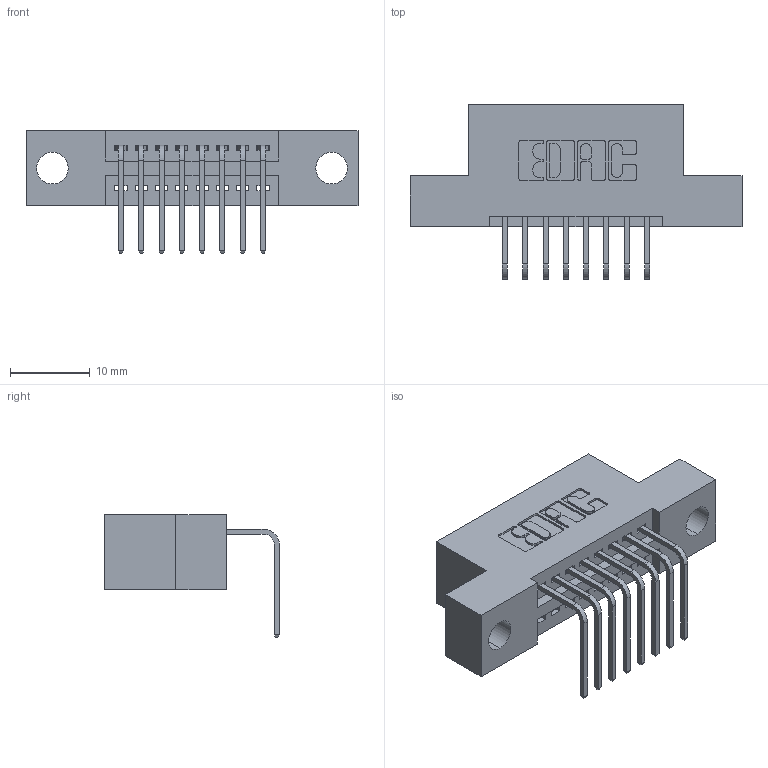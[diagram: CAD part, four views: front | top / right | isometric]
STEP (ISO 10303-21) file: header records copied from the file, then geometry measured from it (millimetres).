
FILE_DESCRIPTION (( 'STEP AP203' ), '1' );
FILE_NAME ('345-008-558-104.STEP', '2021-06-01T16:09:02', ( '' ), ( '' ), 'SwSTEP 2.0', 'SolidWorks 2020', '' );
FILE_SCHEMA (( 'CONFIG_CONTROL_DESIGN' ));
Length unit declared in the file: inch
Products named in the file (3): 345-008-558-104; 345-292-001_558 Tail - 2; 345 Part_Flush Mounting Lugs - 0.156 Dia-TI
Assembly tree (9 placements, depth 2):
  345-008-558-104
    345 Part_Flush Mounting Lugs - 0.156 Dia-TI
    345-292-001_558 Tail - 2  x8
Bounding box: 41.53 x 21.83 x 15.37 mm (x, y, z)
Volume: 3586.7 mm3; surface area: 4303.3 mm2
Topology: 9 solids, 9 shells, 620 faces, 1833 edges, 1210 vertices
Faces by surface type: plane 430, cylinder 190
Entity records: 11101 total; most frequent: CARTESIAN_POINT 1934, ORIENTED_EDGE 1874, DIRECTION 1737, EDGE_CURVE 937, LINE 773, VECTOR 773, VERTEX_POINT 622, AXIS2_PLACEMENT_3D 482
